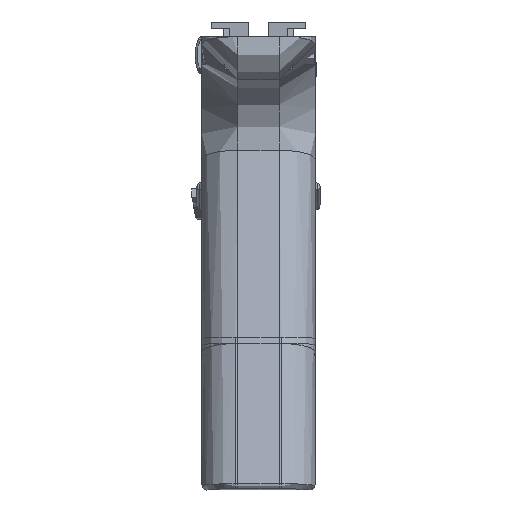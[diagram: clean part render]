
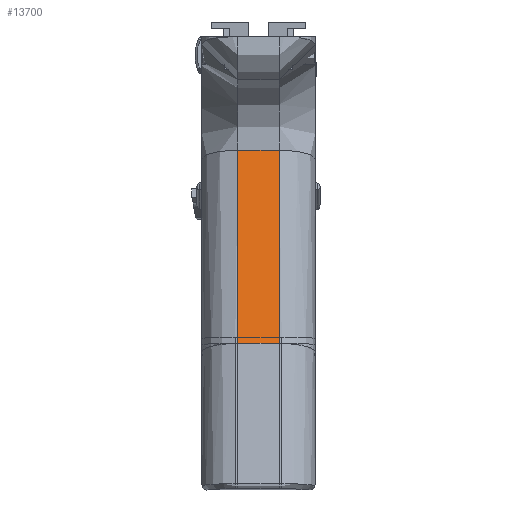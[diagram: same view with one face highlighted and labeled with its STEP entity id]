
A CAD part, front view. The second image highlights one B-rep face of the part: STEP entity #13700.
In plain terms, the highlighted face is planar.
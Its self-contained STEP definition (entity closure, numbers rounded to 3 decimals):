
#990=PLANE('',#14907);
#1597=FACE_OUTER_BOUND('',#2392,.T.);
#2392=EDGE_LOOP('',(#11489,#11490,#11491,#11492));
#3416=LINE('',#22969,#4689);
#3570=LINE('',#23814,#4843);
#3571=LINE('',#23817,#4844);
#3572=LINE('',#23818,#4845);
#4689=VECTOR('',#17385,10.);
#4843=VECTOR('',#17785,10.);
#4844=VECTOR('',#17788,10.);
#4845=VECTOR('',#17789,10.);
#6359=VERTEX_POINT('',#22965);
#6360=VERTEX_POINT('',#22967);
#6495=VERTEX_POINT('',#23792);
#6498=VERTEX_POINT('',#23816);
#8036=EDGE_CURVE('',#6359,#6360,#3416,.T.);
#8260=EDGE_CURVE('',#6359,#6495,#3570,.T.);
#8261=EDGE_CURVE('',#6498,#6360,#3571,.T.);
#8262=EDGE_CURVE('',#6495,#6498,#3572,.T.);
#11489=ORIENTED_EDGE('',*,*,#8261,.F.);
#11490=ORIENTED_EDGE('',*,*,#8262,.F.);
#11491=ORIENTED_EDGE('',*,*,#8260,.F.);
#11492=ORIENTED_EDGE('',*,*,#8036,.T.);
#13700=ADVANCED_FACE('',(#1597),#990,.T.);
#14907=AXIS2_PLACEMENT_3D('',#23815,#17786,#17787);
#17385=DIRECTION('',(0.,-0.249,0.969));
#17785=DIRECTION('',(-1.,0.,0.));
#17786=DIRECTION('center_axis',(0.,-0.969,
-0.249));
#17787=DIRECTION('ref_axis',(0.,-0.249,0.969));
#17788=DIRECTION('',(1.,0.,0.));
#17789=DIRECTION('',(0.,-0.249,0.969));
#22965=CARTESIAN_POINT('',(13.45,-71.634,19.877));
#22967=CARTESIAN_POINT('',(13.45,-83.628,66.536));
#22969=CARTESIAN_POINT('',(13.45,-83.554,66.245));
#23792=CARTESIAN_POINT('',(3.45,-71.634,19.877));
#23814=CARTESIAN_POINT('',(22.175,-71.634,19.877));
#23815=CARTESIAN_POINT('Origin',(22.175,-71.634,19.877));
#23816=CARTESIAN_POINT('',(3.45,-83.628,66.536));
#23817=CARTESIAN_POINT('',(22.175,-83.628,66.536));
#23818=CARTESIAN_POINT('',(3.45,-83.554,66.245));
